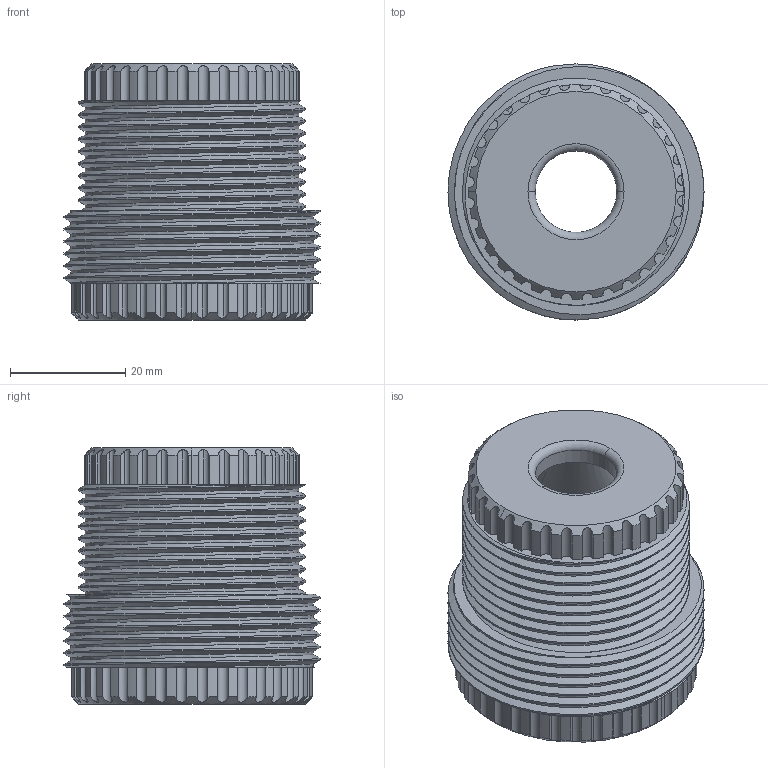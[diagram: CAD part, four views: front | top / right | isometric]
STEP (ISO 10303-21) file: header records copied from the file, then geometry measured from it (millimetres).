
FILE_DESCRIPTION (( 'STEP AP203' ), '1' );
FILE_NAME ('AF-RUGER1022NT-NTMCD-PRT-003-STEP.STEP', '2020-08-29T07:05:03', ( '' ), ( '' ), 'SwSTEP 2.0', 'SolidWorks 2018', '' );
FILE_SCHEMA (( 'CONFIG_CONTROL_DESIGN' ));
Length unit declared in the file: inch
Products named in the file (1): AF-RUGER1022NT-NTMCD-PRT-003-STEP
Bounding box: 44.45 x 44.45 x 44.45 mm (x, y, z)
Volume: 32316.8 mm3; surface area: 13878.1 mm2
Topology: 1 solids, 1 shells, 246 faces, 700 edges, 458 vertices
Faces by surface type: cylinder 206, plane 26, bspline 6, cone 4, torus 4
Entity records: 13104 total; most frequent: CARTESIAN_POINT 6842, ORIENTED_EDGE 1400, DIRECTION 1266, EDGE_CURVE 700, AXIS2_PLACEMENT_3D 529, VERTEX_POINT 458, CIRCLE 288, EDGE_LOOP 250
